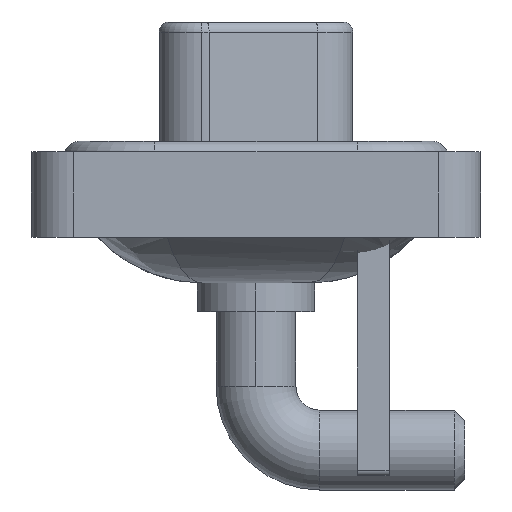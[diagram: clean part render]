
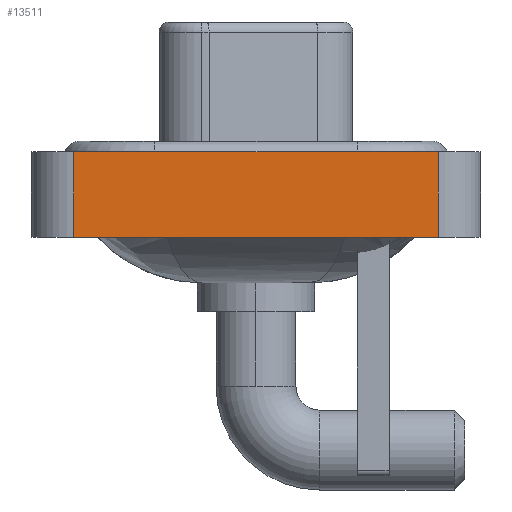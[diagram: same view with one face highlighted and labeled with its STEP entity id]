
A CAD part, left-side view. The second image highlights one B-rep face of the part: STEP entity #13511.
In plain terms, the highlighted planar face has unit normal (-1, 0, 0).
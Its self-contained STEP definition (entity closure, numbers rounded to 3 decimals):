
#355 = EDGE_CURVE ( 'NONE', #10773, #18801, #6225, .T. ) ;
#1056 = VECTOR ( 'NONE', #10913, 1000. ) ;
#1438 = LINE ( 'NONE', #5911, #16616 ) ;
#1999 = CARTESIAN_POINT ( 'NONE',  ( -7.35, -8.55, -3.6 ) ) ;
#2038 = EDGE_CURVE ( 'NONE', #18801, #13599, #5376, .T. ) ;
#2119 = CARTESIAN_POINT ( 'NONE',  ( -7.35, 8.55, -3.6 ) ) ;
#2151 = PLANE ( 'NONE',  #14650 ) ;
#2627 = CARTESIAN_POINT ( 'NONE',  ( -7.35, 8.55, 0.4 ) ) ;
#2898 = EDGE_LOOP ( 'NONE', ( #13244, #9730, #6320, #6403 ) ) ;
#3793 = VECTOR ( 'NONE', #13619, 1000. ) ;
#5376 = LINE ( 'NONE', #11190, #1056 ) ;
#5911 = CARTESIAN_POINT ( 'NONE',  ( -7.35, -8.55, -3.6 ) ) ;
#6225 = LINE ( 'NONE', #2119, #9523 ) ;
#6320 = ORIENTED_EDGE ( 'NONE', *, *, #355, .F. ) ;
#6403 = ORIENTED_EDGE ( 'NONE', *, *, #10349, .T. ) ;
#8063 = DIRECTION ( 'NONE',  ( 0., 0., 1. ) ) ;
#9470 = VERTEX_POINT ( 'NONE', #13362 ) ;
#9481 = CARTESIAN_POINT ( 'NONE',  ( -7.35, -8.55, -3.6 ) ) ;
#9523 = VECTOR ( 'NONE', #12046, 1000. ) ;
#9730 = ORIENTED_EDGE ( 'NONE', *, *, #2038, .F. ) ;
#10349 = EDGE_CURVE ( 'NONE', #10773, #9470, #1438, .T. ) ;
#10773 = VERTEX_POINT ( 'NONE', #17248 ) ;
#10913 = DIRECTION ( 'NONE',  ( 0., -1., 0. ) ) ;
#11190 = CARTESIAN_POINT ( 'NONE',  ( -7.35, -8.55, 0.4 ) ) ;
#12046 = DIRECTION ( 'NONE',  ( 0., 0., 1. ) ) ;
#12546 = LINE ( 'NONE', #1999, #3793 ) ;
#13244 = ORIENTED_EDGE ( 'NONE', *, *, #18095, .T. ) ;
#13362 = CARTESIAN_POINT ( 'NONE',  ( -7.35, -8.55, -3.6 ) ) ;
#13511 = ADVANCED_FACE ( 'NONE', ( #15218 ), #2151, .T. ) ;
#13599 = VERTEX_POINT ( 'NONE', #15588 ) ;
#13619 = DIRECTION ( 'NONE',  ( 0., 0., 1. ) ) ;
#14594 = DIRECTION ( 'NONE',  ( 0., -1., 0. ) ) ;
#14650 = AXIS2_PLACEMENT_3D ( 'NONE', #9481, #15312, #8063 ) ;
#15218 = FACE_OUTER_BOUND ( 'NONE', #2898, .T. ) ;
#15312 = DIRECTION ( 'NONE',  ( -1., 0., 0. ) ) ;
#15588 = CARTESIAN_POINT ( 'NONE',  ( -7.35, -8.55, 0.4 ) ) ;
#16616 = VECTOR ( 'NONE', #14594, 1000. ) ;
#17248 = CARTESIAN_POINT ( 'NONE',  ( -7.35, 8.55, -3.6 ) ) ;
#18095 = EDGE_CURVE ( 'NONE', #9470, #13599, #12546, .T. ) ;
#18801 = VERTEX_POINT ( 'NONE', #2627 ) ;
